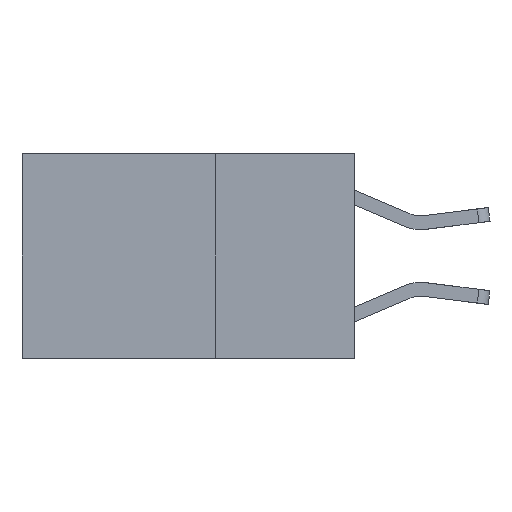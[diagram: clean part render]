
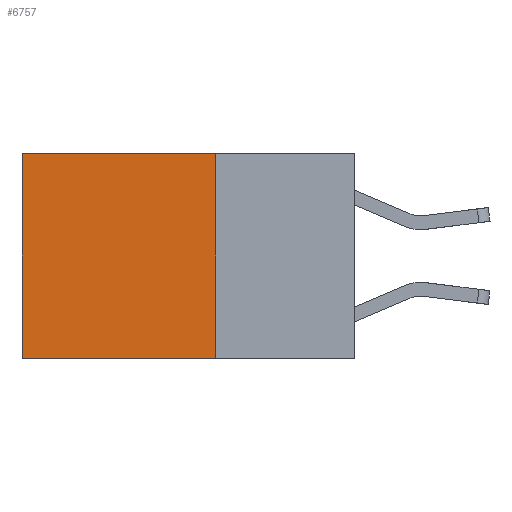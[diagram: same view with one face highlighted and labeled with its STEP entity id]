
A CAD part, left-side view. The second image highlights one B-rep face of the part: STEP entity #6757.
In plain terms, the highlighted planar face has unit normal (-1, 0, 0).
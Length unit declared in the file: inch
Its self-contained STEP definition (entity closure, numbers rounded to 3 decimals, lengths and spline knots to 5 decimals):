
#696 = VERTEX_POINT ( 'NONE', #6604 ) ;
#932 = DIRECTION ( 'NONE',  ( 0., 0., -1. ) ) ;
#960 = EDGE_LOOP ( 'NONE', ( #1313, #6561, #7386, #8360 ) ) ;
#1158 = DIRECTION ( 'NONE',  ( 0., 0., -1. ) ) ;
#1313 = ORIENTED_EDGE ( 'NONE', *, *, #8323, .T. ) ;
#1361 = AXIS2_PLACEMENT_3D ( 'NONE', #4853, #7708, #2976 ) ;
#1364 = EDGE_CURVE ( 'NONE', #8329, #4321, #6887, .T. ) ;
#1736 = EDGE_CURVE ( 'NONE', #696, #8329, #7769, .T. ) ;
#2292 = DIRECTION ( 'NONE',  ( 0., 1., 0. ) ) ;
#2976 = DIRECTION ( 'NONE',  ( 0., 0., -1. ) ) ;
#2990 = CARTESIAN_POINT ( 'NONE',  ( 0.2625, 0.25, -0.37 ) ) ;
#3192 = VERTEX_POINT ( 'NONE', #5074 ) ;
#3719 = CARTESIAN_POINT ( 'NONE',  ( 0.2625, 0.25, 0. ) ) ;
#4207 = LINE ( 'NONE', #5073, #5244 ) ;
#4321 = VERTEX_POINT ( 'NONE', #5171 ) ;
#4853 = CARTESIAN_POINT ( 'NONE',  ( 0.2625, 0.25, 0. ) ) ;
#5073 = CARTESIAN_POINT ( 'NONE',  ( 0.2625, 0.25, 0. ) ) ;
#5074 = CARTESIAN_POINT ( 'NONE',  ( 0.2625, 0.6, 0. ) ) ;
#5171 = CARTESIAN_POINT ( 'NONE',  ( 0.2625, 0.6, -0.37 ) ) ;
#5244 = VECTOR ( 'NONE', #2292, 39.37008 ) ;
#5900 = EDGE_CURVE ( 'NONE', #696, #3192, #4207, .T. ) ;
#6215 = PLANE ( 'NONE',  #1361 ) ;
#6366 = CARTESIAN_POINT ( 'NONE',  ( 0.2625, 0.25, -0.37 ) ) ;
#6561 = ORIENTED_EDGE ( 'NONE', *, *, #1364, .F. ) ;
#6604 = CARTESIAN_POINT ( 'NONE',  ( 0.2625, 0.25, 0. ) ) ;
#6757 = ADVANCED_FACE ( 'NONE', ( #8231 ), #6215, .F. ) ;
#6887 = LINE ( 'NONE', #2990, #8136 ) ;
#7386 = ORIENTED_EDGE ( 'NONE', *, *, #1736, .F. ) ;
#7708 = DIRECTION ( 'NONE',  ( 1., 0., 0. ) ) ;
#7733 = LINE ( 'NONE', #8538, #8528 ) ;
#7769 = LINE ( 'NONE', #3719, #8010 ) ;
#8010 = VECTOR ( 'NONE', #932, 39.37008 ) ;
#8136 = VECTOR ( 'NONE', #8250, 39.37008 ) ;
#8231 = FACE_OUTER_BOUND ( 'NONE', #960, .T. ) ;
#8250 = DIRECTION ( 'NONE',  ( 0., 1., 0. ) ) ;
#8323 = EDGE_CURVE ( 'NONE', #3192, #4321, #7733, .T. ) ;
#8329 = VERTEX_POINT ( 'NONE', #6366 ) ;
#8360 = ORIENTED_EDGE ( 'NONE', *, *, #5900, .T. ) ;
#8528 = VECTOR ( 'NONE', #1158, 39.37008 ) ;
#8538 = CARTESIAN_POINT ( 'NONE',  ( 0.2625, 0.6, 0. ) ) ;
